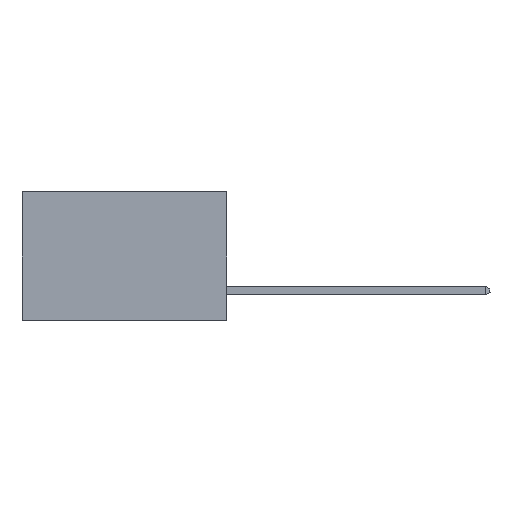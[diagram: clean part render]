
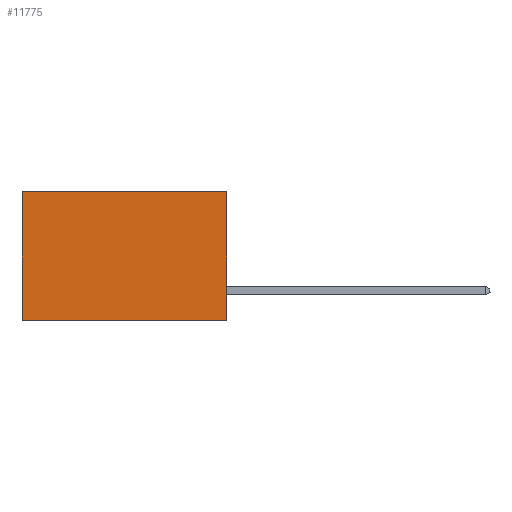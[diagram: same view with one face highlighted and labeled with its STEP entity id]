
A CAD part, left-side view. The second image highlights one B-rep face of the part: STEP entity #11775.
In plain terms, the highlighted planar face has unit normal (-1, 0, 0).
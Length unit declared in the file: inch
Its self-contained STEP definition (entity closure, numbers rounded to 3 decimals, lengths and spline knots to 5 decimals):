
#308 = VERTEX_POINT ( 'NONE', #5615 ) ;
#344 = PLANE ( 'NONE',  #8235 ) ;
#785 = VERTEX_POINT ( 'NONE', #17980 ) ;
#1035 = VERTEX_POINT ( 'NONE', #6705 ) ;
#1608 = FACE_OUTER_BOUND ( 'NONE', #3127, .T. ) ;
#1872 = DIRECTION ( 'NONE',  ( 0., 1., 0. ) ) ;
#1925 = EDGE_CURVE ( 'NONE', #1035, #3063, #4819, .T. ) ;
#2217 = CARTESIAN_POINT ( 'NONE',  ( 0.277, 0., -0.37 ) ) ;
#2608 = VECTOR ( 'NONE', #4767, 39.37008 ) ;
#3063 = VERTEX_POINT ( 'NONE', #18571 ) ;
#3127 = EDGE_LOOP ( 'NONE', ( #13091, #7486, #12563, #8585 ) ) ;
#3411 = DIRECTION ( 'NONE',  ( 1., 0., 0. ) ) ;
#4315 = CARTESIAN_POINT ( 'NONE',  ( 0.277, 0.59, -0.37 ) ) ;
#4333 = VECTOR ( 'NONE', #1872, 39.37008 ) ;
#4564 = EDGE_CURVE ( 'NONE', #308, #1035, #7106, .T. ) ;
#4767 = DIRECTION ( 'NONE',  ( 0., 0., -1. ) ) ;
#4807 = VECTOR ( 'NONE', #17906, 39.37008 ) ;
#4819 = LINE ( 'NONE', #8723, #4333 ) ;
#5615 = CARTESIAN_POINT ( 'NONE',  ( 0.277, 0., 0. ) ) ;
#5818 = LINE ( 'NONE', #8642, #17390 ) ;
#6705 = CARTESIAN_POINT ( 'NONE',  ( 0.277, 0., -0.37 ) ) ;
#7106 = LINE ( 'NONE', #2217, #2608 ) ;
#7486 = ORIENTED_EDGE ( 'NONE', *, *, #1925, .F. ) ;
#8235 = AXIS2_PLACEMENT_3D ( 'NONE', #12404, #3411, #13931 ) ;
#8585 = ORIENTED_EDGE ( 'NONE', *, *, #19248, .T. ) ;
#8642 = CARTESIAN_POINT ( 'NONE',  ( 0.277, 0., 0. ) ) ;
#8723 = CARTESIAN_POINT ( 'NONE',  ( 0.277, 0., -0.37 ) ) ;
#8823 = LINE ( 'NONE', #4315, #4807 ) ;
#10132 = DIRECTION ( 'NONE',  ( 0., 1., 0. ) ) ;
#11775 = ADVANCED_FACE ( 'NONE', ( #1608 ), #344, .F. ) ;
#12404 = CARTESIAN_POINT ( 'NONE',  ( 0.277, 0., -0.37 ) ) ;
#12563 = ORIENTED_EDGE ( 'NONE', *, *, #4564, .F. ) ;
#13091 = ORIENTED_EDGE ( 'NONE', *, *, #16951, .T. ) ;
#13931 = DIRECTION ( 'NONE',  ( 0., 0., -1. ) ) ;
#16951 = EDGE_CURVE ( 'NONE', #785, #3063, #8823, .T. ) ;
#17390 = VECTOR ( 'NONE', #10132, 39.37008 ) ;
#17906 = DIRECTION ( 'NONE',  ( 0., 0., -1. ) ) ;
#17980 = CARTESIAN_POINT ( 'NONE',  ( 0.277, 0.59, 0. ) ) ;
#18571 = CARTESIAN_POINT ( 'NONE',  ( 0.277, 0.59, -0.37 ) ) ;
#19248 = EDGE_CURVE ( 'NONE', #308, #785, #5818, .T. ) ;
